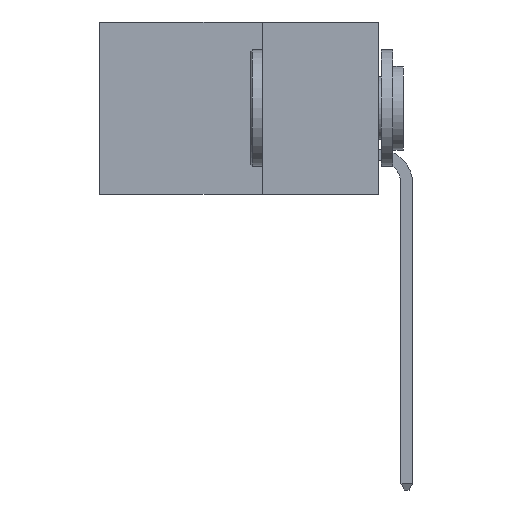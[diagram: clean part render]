
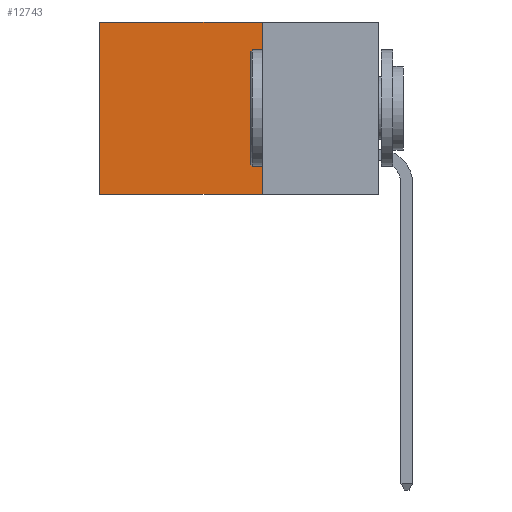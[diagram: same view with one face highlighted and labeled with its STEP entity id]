
A CAD part, left-side view. The second image highlights one B-rep face of the part: STEP entity #12743.
In plain terms, the highlighted planar face has unit normal (-1, 0, 0).
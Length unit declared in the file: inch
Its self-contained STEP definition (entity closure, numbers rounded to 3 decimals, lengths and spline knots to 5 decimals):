
#1236 = EDGE_CURVE ( 'NONE', #1447, #19526, #19601, .T. ) ;
#1447 = VERTEX_POINT ( 'NONE', #14963 ) ;
#1797 = VECTOR ( 'NONE', #6393, 39.37008 ) ;
#3608 = CARTESIAN_POINT ( 'NONE',  ( 0.2615, 0.25, -0.37 ) ) ;
#3725 = VECTOR ( 'NONE', #13596, 39.37008 ) ;
#4912 = EDGE_CURVE ( 'NONE', #17949, #1447, #16241, .T. ) ;
#5273 = CARTESIAN_POINT ( 'NONE',  ( 0.2615, 0.6, 0. ) ) ;
#5965 = CARTESIAN_POINT ( 'NONE',  ( 0.2615, 0.25, -0.37 ) ) ;
#6393 = DIRECTION ( 'NONE',  ( 0., 0., -1. ) ) ;
#6778 = EDGE_LOOP ( 'NONE', ( #16930, #19992, #9058, #8871 ) ) ;
#7558 = DIRECTION ( 'NONE',  ( 0., 0., -1. ) ) ;
#8871 = ORIENTED_EDGE ( 'NONE', *, *, #12269, .T. ) ;
#9058 = ORIENTED_EDGE ( 'NONE', *, *, #4912, .F. ) ;
#9941 = VERTEX_POINT ( 'NONE', #5273 ) ;
#10829 = CARTESIAN_POINT ( 'NONE',  ( 0.2615, 0.6, -0.37 ) ) ;
#12223 = AXIS2_PLACEMENT_3D ( 'NONE', #5965, #16986, #7558 ) ;
#12269 = EDGE_CURVE ( 'NONE', #17949, #9941, #19970, .T. ) ;
#12279 = PLANE ( 'NONE',  #12223 ) ;
#12716 = CARTESIAN_POINT ( 'NONE',  ( 0.2615, 0.25, 0. ) ) ;
#12722 = CARTESIAN_POINT ( 'NONE',  ( 0.2615, 0.6, -0.37 ) ) ;
#12743 = ADVANCED_FACE ( 'NONE', ( #15537 ), #12279, .F. ) ;
#13596 = DIRECTION ( 'NONE',  ( 0., 0., -1. ) ) ;
#13862 = CARTESIAN_POINT ( 'NONE',  ( 0.2615, 0.25, -0.37 ) ) ;
#13864 = LINE ( 'NONE', #12722, #1797 ) ;
#14309 = DIRECTION ( 'NONE',  ( 0., 1., 0. ) ) ;
#14880 = DIRECTION ( 'NONE',  ( 0., 1., 0. ) ) ;
#14963 = CARTESIAN_POINT ( 'NONE',  ( 0.2615, 0.25, -0.37 ) ) ;
#15537 = FACE_OUTER_BOUND ( 'NONE', #6778, .T. ) ;
#15931 = EDGE_CURVE ( 'NONE', #9941, #19526, #13864, .T. ) ;
#16039 = VECTOR ( 'NONE', #14309, 39.37008 ) ;
#16128 = VECTOR ( 'NONE', #14880, 39.37008 ) ;
#16241 = LINE ( 'NONE', #13862, #3725 ) ;
#16930 = ORIENTED_EDGE ( 'NONE', *, *, #15931, .T. ) ;
#16986 = DIRECTION ( 'NONE',  ( 1., 0., 0. ) ) ;
#17949 = VERTEX_POINT ( 'NONE', #19258 ) ;
#19258 = CARTESIAN_POINT ( 'NONE',  ( 0.2615, 0.25, 0. ) ) ;
#19526 = VERTEX_POINT ( 'NONE', #10829 ) ;
#19601 = LINE ( 'NONE', #3608, #16128 ) ;
#19970 = LINE ( 'NONE', #12716, #16039 ) ;
#19992 = ORIENTED_EDGE ( 'NONE', *, *, #1236, .F. ) ;
